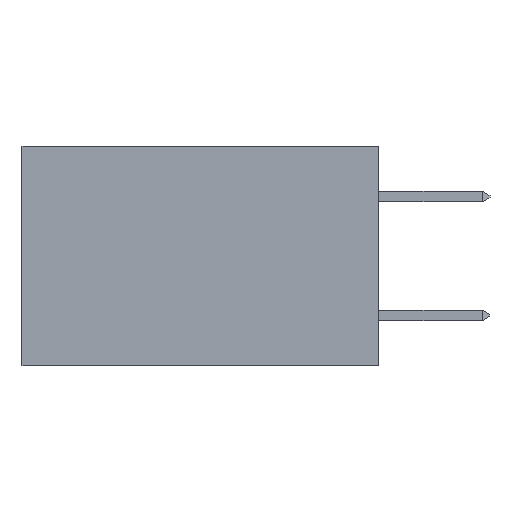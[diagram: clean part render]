
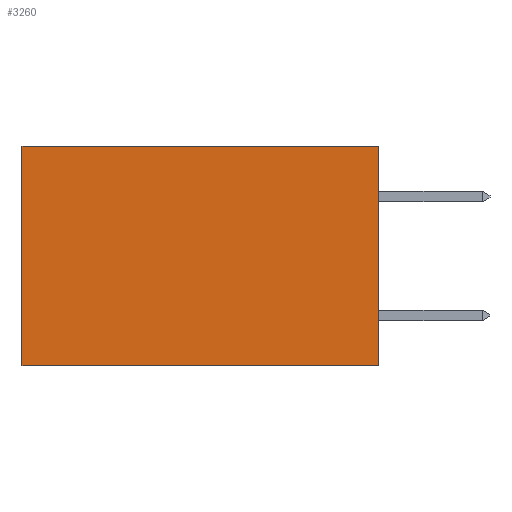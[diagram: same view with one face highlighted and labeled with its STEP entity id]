
A CAD part, left-side view. The second image highlights one B-rep face of the part: STEP entity #3260.
In plain terms, the highlighted planar face has unit normal (-1, 0, 0).
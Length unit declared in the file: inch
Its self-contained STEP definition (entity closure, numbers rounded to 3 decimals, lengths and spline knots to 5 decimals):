
#276 = LINE ( 'NONE', #997, #7816 ) ;
#733 = VECTOR ( 'NONE', #943, 39.37008 ) ;
#943 = DIRECTION ( 'NONE',  ( 0., 1., 0. ) ) ;
#975 = LINE ( 'NONE', #9012, #733 ) ;
#997 = CARTESIAN_POINT ( 'NONE',  ( 0.298, 0., 0. ) ) ;
#1113 = VERTEX_POINT ( 'NONE', #2221 ) ;
#1489 = DIRECTION ( 'NONE',  ( 0., 0., -1. ) ) ;
#1512 = EDGE_CURVE ( 'NONE', #1693, #1113, #6972, .T. ) ;
#1693 = VERTEX_POINT ( 'NONE', #7101 ) ;
#1847 = EDGE_CURVE ( 'NONE', #6202, #8229, #8209, .T. ) ;
#2221 = CARTESIAN_POINT ( 'NONE',  ( 0.298, 0.6, -0.37 ) ) ;
#3101 = CARTESIAN_POINT ( 'NONE',  ( 0.298, 0., 0. ) ) ;
#3260 = ADVANCED_FACE ( 'NONE', ( #7911 ), #4922, .F. ) ;
#3470 = EDGE_LOOP ( 'NONE', ( #3760, #3785, #4211, #4316 ) ) ;
#3760 = ORIENTED_EDGE ( 'NONE', *, *, #1512, .T. ) ;
#3785 = ORIENTED_EDGE ( 'NONE', *, *, #4880, .F. ) ;
#4211 = ORIENTED_EDGE ( 'NONE', *, *, #1847, .F. ) ;
#4316 = ORIENTED_EDGE ( 'NONE', *, *, #4436, .T. ) ;
#4436 = EDGE_CURVE ( 'NONE', #6202, #1693, #276, .T. ) ;
#4578 = CARTESIAN_POINT ( 'NONE',  ( 0.298, 0., 0. ) ) ;
#4794 = AXIS2_PLACEMENT_3D ( 'NONE', #5587, #4802, #5167 ) ;
#4802 = DIRECTION ( 'NONE',  ( 1., 0., 0. ) ) ;
#4880 = EDGE_CURVE ( 'NONE', #8229, #1113, #975, .T. ) ;
#4909 = CARTESIAN_POINT ( 'NONE',  ( 0.298, 0., -0.37 ) ) ;
#4922 = PLANE ( 'NONE',  #4794 ) ;
#5167 = DIRECTION ( 'NONE',  ( 0., 0., -1. ) ) ;
#5587 = CARTESIAN_POINT ( 'NONE',  ( 0.298, 0., 0. ) ) ;
#5679 = DIRECTION ( 'NONE',  ( 0., 0., -1. ) ) ;
#6202 = VERTEX_POINT ( 'NONE', #3101 ) ;
#6342 = CARTESIAN_POINT ( 'NONE',  ( 0.298, 0.6, 0. ) ) ;
#6443 = VECTOR ( 'NONE', #1489, 39.37008 ) ;
#6972 = LINE ( 'NONE', #6342, #8503 ) ;
#7101 = CARTESIAN_POINT ( 'NONE',  ( 0.298, 0.6, 0. ) ) ;
#7723 = DIRECTION ( 'NONE',  ( 0., 1., 0. ) ) ;
#7816 = VECTOR ( 'NONE', #7723, 39.37008 ) ;
#7911 = FACE_OUTER_BOUND ( 'NONE', #3470, .T. ) ;
#8209 = LINE ( 'NONE', #4578, #6443 ) ;
#8229 = VERTEX_POINT ( 'NONE', #4909 ) ;
#8503 = VECTOR ( 'NONE', #5679, 39.37008 ) ;
#9012 = CARTESIAN_POINT ( 'NONE',  ( 0.298, 0., -0.37 ) ) ;
